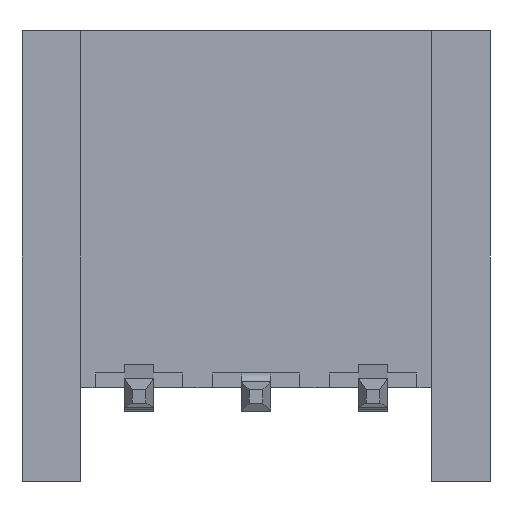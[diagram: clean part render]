
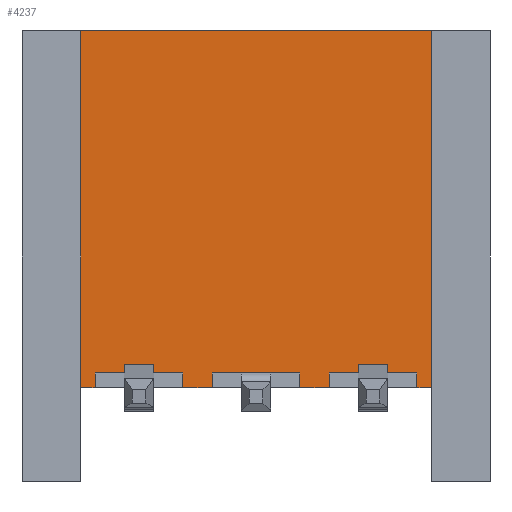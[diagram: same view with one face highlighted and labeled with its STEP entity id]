
A CAD part, front view. The second image highlights one B-rep face of the part: STEP entity #4237.
In plain terms, the highlighted planar face has unit normal (0, -1, 0).
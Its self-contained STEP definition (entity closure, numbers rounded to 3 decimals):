
#42 = VERTEX_POINT ( 'NONE', #1627 ) ;
#69 = CARTESIAN_POINT ( 'NONE',  ( 0.75, -2.9, 0.25 ) ) ;
#82 = VERTEX_POINT ( 'NONE', #321 ) ;
#88 = VERTEX_POINT ( 'NONE', #981 ) ;
#92 = CARTESIAN_POINT ( 'NONE',  ( -0.75, -2.9, 0.25 ) ) ;
#118 = LINE ( 'NONE', #2345, #3847 ) ;
#124 = ORIENTED_EDGE ( 'NONE', *, *, #4217, .F. ) ;
#180 = DIRECTION ( 'NONE',  ( 1., 0., 0. ) ) ;
#212 = CARTESIAN_POINT ( 'NONE',  ( 5., -2.9, -1.6 ) ) ;
#219 = EDGE_CURVE ( 'NONE', #3987, #42, #588, .T. ) ;
#280 = LINE ( 'NONE', #2099, #2706 ) ;
#289 = VERTEX_POINT ( 'NONE', #302 ) ;
#300 = VECTOR ( 'NONE', #180, 1000. ) ;
#302 = CARTESIAN_POINT ( 'NONE',  ( -1., -2.9, 0. ) ) ;
#317 = VERTEX_POINT ( 'NONE', #403 ) ;
#321 = CARTESIAN_POINT ( 'NONE',  ( 5., -2.9, 0. ) ) ;
#331 = LINE ( 'NONE', #3257, #906 ) ;
#338 = EDGE_LOOP ( 'NONE', ( #2414, #3730, #3019, #3970, #2258, #1327, #4001, #3156, #2872, #1470, #124, #1227, #2813, #1992, #353, #1609 ) ) ;
#342 = LINE ( 'NONE', #4018, #1176 ) ;
#343 = DIRECTION ( 'NONE',  ( -1., 0., 0. ) ) ;
#353 = ORIENTED_EDGE ( 'NONE', *, *, #3181, .T. ) ;
#376 = LINE ( 'NONE', #2338, #1671 ) ;
#403 = CARTESIAN_POINT ( 'NONE',  ( -0.75, -2.9, 0. ) ) ;
#433 = DIRECTION ( 'NONE',  ( 0., 0., 1. ) ) ;
#500 = VERTEX_POINT ( 'NONE', #1735 ) ;
#502 = VECTOR ( 'NONE', #3408, 1000. ) ;
#577 = CARTESIAN_POINT ( 'NONE',  ( 1.25, -2.9, 0. ) ) ;
#588 = LINE ( 'NONE', #3606, #2958 ) ;
#723 = DIRECTION ( 'NONE',  ( 0., 0., 1. ) ) ;
#740 = EDGE_CURVE ( 'NONE', #1958, #82, #3885, .T. ) ;
#777 = CARTESIAN_POINT ( 'NONE',  ( -1., -2.9, -1.6 ) ) ;
#804 = VERTEX_POINT ( 'NONE', #1634 ) ;
#906 = VECTOR ( 'NONE', #4269, 1000. ) ;
#981 = CARTESIAN_POINT ( 'NONE',  ( 0.75, -2.9, 0.25 ) ) ;
#1036 = DIRECTION ( 'NONE',  ( 0., 0., -1. ) ) ;
#1093 = EDGE_CURVE ( 'NONE', #804, #3987, #1561, .T. ) ;
#1149 = CARTESIAN_POINT ( 'NONE',  ( 4.75, -2.9, 0.25 ) ) ;
#1176 = VECTOR ( 'NONE', #1460, 1000. ) ;
#1227 = ORIENTED_EDGE ( 'NONE', *, *, #3666, .F. ) ;
#1327 = ORIENTED_EDGE ( 'NONE', *, *, #2521, .F. ) ;
#1431 = LINE ( 'NONE', #69, #2669 ) ;
#1439 = VECTOR ( 'NONE', #4083, 1000. ) ;
#1460 = DIRECTION ( 'NONE',  ( 0., 0., -1. ) ) ;
#1470 = ORIENTED_EDGE ( 'NONE', *, *, #2407, .F. ) ;
#1561 = LINE ( 'NONE', #3056, #4075 ) ;
#1565 = VECTOR ( 'NONE', #3913, 1000. ) ;
#1581 = CARTESIAN_POINT ( 'NONE',  ( 4.75, -2.9, 0.25 ) ) ;
#1592 = CARTESIAN_POINT ( 'NONE',  ( 4.75, -2.9, 0. ) ) ;
#1609 = ORIENTED_EDGE ( 'NONE', *, *, #2469, .F. ) ;
#1627 = CARTESIAN_POINT ( 'NONE',  ( 1.25, -2.9, 0.25 ) ) ;
#1631 = CARTESIAN_POINT ( 'NONE',  ( 5., -2.9, 6.1 ) ) ;
#1634 = CARTESIAN_POINT ( 'NONE',  ( 2.75, -2.9, 0. ) ) ;
#1667 = VECTOR ( 'NONE', #1929, 1000. ) ;
#1671 = VECTOR ( 'NONE', #2683, 1000. ) ;
#1691 = PLANE ( 'NONE',  #4155 ) ;
#1734 = VERTEX_POINT ( 'NONE', #2825 ) ;
#1735 = CARTESIAN_POINT ( 'NONE',  ( 3.25, -2.9, 0. ) ) ;
#1773 = LINE ( 'NONE', #212, #3418 ) ;
#1862 = EDGE_CURVE ( 'NONE', #804, #500, #2630, .T. ) ;
#1911 = VERTEX_POINT ( 'NONE', #3485 ) ;
#1929 = DIRECTION ( 'NONE',  ( -1., 0., 0. ) ) ;
#1958 = VERTEX_POINT ( 'NONE', #1592 ) ;
#1979 = VERTEX_POINT ( 'NONE', #577 ) ;
#1992 = ORIENTED_EDGE ( 'NONE', *, *, #4189, .T. ) ;
#2052 = CARTESIAN_POINT ( 'NONE',  ( 1.25, -2.9, 0.25 ) ) ;
#2064 = EDGE_CURVE ( 'NONE', #289, #317, #2232, .T. ) ;
#2090 = DIRECTION ( 'NONE',  ( 0., 0., 1. ) ) ;
#2099 = CARTESIAN_POINT ( 'NONE',  ( 4.75, -2.9, 0.25 ) ) ;
#2120 = CARTESIAN_POINT ( 'NONE',  ( 0.75, -2.9, 0. ) ) ;
#2139 = VERTEX_POINT ( 'NONE', #1631 ) ;
#2232 = LINE ( 'NONE', #3579, #3285 ) ;
#2239 = EDGE_CURVE ( 'NONE', #2786, #1979, #4056, .T. ) ;
#2258 = ORIENTED_EDGE ( 'NONE', *, *, #2239, .T. ) ;
#2314 = VERTEX_POINT ( 'NONE', #1149 ) ;
#2338 = CARTESIAN_POINT ( 'NONE',  ( -0.75, -2.9, 0.25 ) ) ;
#2345 = CARTESIAN_POINT ( 'NONE',  ( 0.75, -2.9, 0.25 ) ) ;
#2407 = EDGE_CURVE ( 'NONE', #1911, #500, #342, .T. ) ;
#2414 = ORIENTED_EDGE ( 'NONE', *, *, #2064, .T. ) ;
#2415 = CARTESIAN_POINT ( 'NONE',  ( 2.75, -2.9, 0.25 ) ) ;
#2417 = CARTESIAN_POINT ( 'NONE',  ( 6., -2.9, 0. ) ) ;
#2454 = VERTEX_POINT ( 'NONE', #92 ) ;
#2469 = EDGE_CURVE ( 'NONE', #289, #1734, #3335, .T. ) ;
#2521 = EDGE_CURVE ( 'NONE', #42, #1979, #2673, .T. ) ;
#2630 = LINE ( 'NONE', #3815, #300 ) ;
#2650 = EDGE_CURVE ( 'NONE', #2786, #88, #1431, .T. ) ;
#2651 = LINE ( 'NONE', #1581, #1667 ) ;
#2669 = VECTOR ( 'NONE', #723, 1000. ) ;
#2673 = LINE ( 'NONE', #2052, #4252 ) ;
#2683 = DIRECTION ( 'NONE',  ( 0., 0., -1. ) ) ;
#2706 = VECTOR ( 'NONE', #433, 1000. ) ;
#2786 = VERTEX_POINT ( 'NONE', #2120 ) ;
#2813 = ORIENTED_EDGE ( 'NONE', *, *, #740, .T. ) ;
#2825 = CARTESIAN_POINT ( 'NONE',  ( -1., -2.9, 6.1 ) ) ;
#2872 = ORIENTED_EDGE ( 'NONE', *, *, #1862, .T. ) ;
#2958 = VECTOR ( 'NONE', #3951, 1000. ) ;
#3019 = ORIENTED_EDGE ( 'NONE', *, *, #3280, .F. ) ;
#3022 = DIRECTION ( 'NONE',  ( 0., 1., 0. ) ) ;
#3056 = CARTESIAN_POINT ( 'NONE',  ( 2.75, -2.9, 0.25 ) ) ;
#3113 = FACE_OUTER_BOUND ( 'NONE', #338, .T. ) ;
#3156 = ORIENTED_EDGE ( 'NONE', *, *, #1093, .F. ) ;
#3181 = EDGE_CURVE ( 'NONE', #2139, #1734, #331, .T. ) ;
#3238 = DIRECTION ( 'NONE',  ( 0., 0., 1. ) ) ;
#3257 = CARTESIAN_POINT ( 'NONE',  ( 5., -2.9, 6.1 ) ) ;
#3272 = DIRECTION ( 'NONE',  ( 1., 0., 0. ) ) ;
#3280 = EDGE_CURVE ( 'NONE', #88, #2454, #118, .T. ) ;
#3285 = VECTOR ( 'NONE', #3272, 1000. ) ;
#3335 = LINE ( 'NONE', #777, #502 ) ;
#3408 = DIRECTION ( 'NONE',  ( 0., 0., 1. ) ) ;
#3418 = VECTOR ( 'NONE', #3238, 1000. ) ;
#3485 = CARTESIAN_POINT ( 'NONE',  ( 3.25, -2.9, 0.25 ) ) ;
#3557 = CARTESIAN_POINT ( 'NONE',  ( 6., -2.9, 0. ) ) ;
#3579 = CARTESIAN_POINT ( 'NONE',  ( 6., -2.9, 0. ) ) ;
#3606 = CARTESIAN_POINT ( 'NONE',  ( 2.75, -2.9, 0.25 ) ) ;
#3645 = DIRECTION ( 'NONE',  ( -1., 0., 0. ) ) ;
#3660 = EDGE_CURVE ( 'NONE', #2454, #317, #376, .T. ) ;
#3666 = EDGE_CURVE ( 'NONE', #1958, #2314, #280, .T. ) ;
#3730 = ORIENTED_EDGE ( 'NONE', *, *, #3660, .F. ) ;
#3815 = CARTESIAN_POINT ( 'NONE',  ( 6., -2.9, 0. ) ) ;
#3847 = VECTOR ( 'NONE', #343, 1000. ) ;
#3885 = LINE ( 'NONE', #3557, #1565 ) ;
#3913 = DIRECTION ( 'NONE',  ( 1., 0., 0. ) ) ;
#3951 = DIRECTION ( 'NONE',  ( -1., 0., 0. ) ) ;
#3970 = ORIENTED_EDGE ( 'NONE', *, *, #2650, .F. ) ;
#3987 = VERTEX_POINT ( 'NONE', #2415 ) ;
#3994 = CARTESIAN_POINT ( 'NONE',  ( 5., -2.9, -1.6 ) ) ;
#4001 = ORIENTED_EDGE ( 'NONE', *, *, #219, .F. ) ;
#4018 = CARTESIAN_POINT ( 'NONE',  ( 3.25, -2.9, 0.25 ) ) ;
#4056 = LINE ( 'NONE', #2417, #1439 ) ;
#4075 = VECTOR ( 'NONE', #2090, 1000. ) ;
#4083 = DIRECTION ( 'NONE',  ( 1., 0., 0. ) ) ;
#4155 = AXIS2_PLACEMENT_3D ( 'NONE', #3994, #3022, #3645 ) ;
#4189 = EDGE_CURVE ( 'NONE', #82, #2139, #1773, .T. ) ;
#4217 = EDGE_CURVE ( 'NONE', #2314, #1911, #2651, .T. ) ;
#4237 = ADVANCED_FACE ( 'NONE', ( #3113 ), #1691, .F. ) ;
#4252 = VECTOR ( 'NONE', #1036, 1000. ) ;
#4269 = DIRECTION ( 'NONE',  ( -1., 0., 0. ) ) ;
